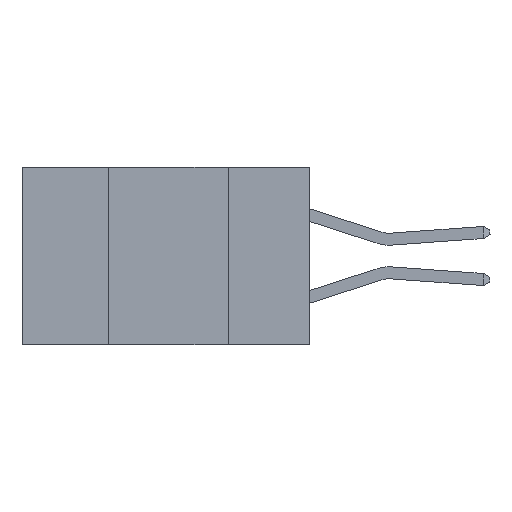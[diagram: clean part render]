
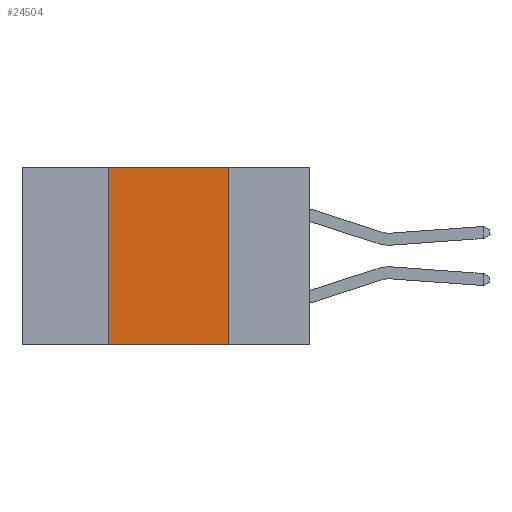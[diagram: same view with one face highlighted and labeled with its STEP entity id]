
A CAD part, left-side view. The second image highlights one B-rep face of the part: STEP entity #24504.
In plain terms, the highlighted planar face has unit normal (-1, 0, 0).
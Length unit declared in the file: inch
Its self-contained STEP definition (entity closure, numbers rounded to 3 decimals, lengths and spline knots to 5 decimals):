
#2264 = CARTESIAN_POINT ( 'NONE',  ( 0., 0.17, -0.37 ) ) ;
#2955 = FACE_OUTER_BOUND ( 'NONE', #8184, .T. ) ;
#3680 = VERTEX_POINT ( 'NONE', #21268 ) ;
#4613 = LINE ( 'NONE', #9639, #26238 ) ;
#5525 = PLANE ( 'NONE',  #18120 ) ;
#5615 = DIRECTION ( 'NONE',  ( 1., 0., 0. ) ) ;
#5854 = VERTEX_POINT ( 'NONE', #12949 ) ;
#7232 = DIRECTION ( 'NONE',  ( 0., -1., 0. ) ) ;
#7438 = ORIENTED_EDGE ( 'NONE', *, *, #27174, .T. ) ;
#7776 = EDGE_CURVE ( 'NONE', #5854, #3680, #4613, .T. ) ;
#8184 = EDGE_LOOP ( 'NONE', ( #24159, #22562, #12964, #7438 ) ) ;
#8770 = CARTESIAN_POINT ( 'NONE',  ( 0., 0.17, 0. ) ) ;
#9639 = CARTESIAN_POINT ( 'NONE',  ( 0., 0.42, -0.37 ) ) ;
#12634 = LINE ( 'NONE', #25622, #23812 ) ;
#12949 = CARTESIAN_POINT ( 'NONE',  ( 0., 0.42, -0.37 ) ) ;
#12964 = ORIENTED_EDGE ( 'NONE', *, *, #7776, .F. ) ;
#12987 = LINE ( 'NONE', #21781, #23513 ) ;
#14763 = VECTOR ( 'NONE', #7232, 39.37008 ) ;
#15152 = DIRECTION ( 'NONE',  ( 0., 0., -1. ) ) ;
#15993 = EDGE_CURVE ( 'NONE', #3680, #23481, #25927, .T. ) ;
#16129 = DIRECTION ( 'NONE',  ( 0., 0., 1. ) ) ;
#18120 = AXIS2_PLACEMENT_3D ( 'NONE', #26494, #5615, #20287 ) ;
#18886 = VERTEX_POINT ( 'NONE', #2264 ) ;
#19006 = EDGE_CURVE ( 'NONE', #23481, #18886, #12634, .T. ) ;
#20287 = DIRECTION ( 'NONE',  ( 0., 0., -1. ) ) ;
#21268 = CARTESIAN_POINT ( 'NONE',  ( 0., 0.42, 0. ) ) ;
#21781 = CARTESIAN_POINT ( 'NONE',  ( 0., 0.6, -0.37 ) ) ;
#21898 = CARTESIAN_POINT ( 'NONE',  ( 0., 0.6, 0. ) ) ;
#22562 = ORIENTED_EDGE ( 'NONE', *, *, #15993, .F. ) ;
#23481 = VERTEX_POINT ( 'NONE', #8770 ) ;
#23513 = VECTOR ( 'NONE', #23899, 39.37008 ) ;
#23812 = VECTOR ( 'NONE', #15152, 39.37008 ) ;
#23899 = DIRECTION ( 'NONE',  ( 0., -1., 0. ) ) ;
#24159 = ORIENTED_EDGE ( 'NONE', *, *, #19006, .F. ) ;
#24504 = ADVANCED_FACE ( 'NONE', ( #2955 ), #5525, .F. ) ;
#25622 = CARTESIAN_POINT ( 'NONE',  ( 0., 0.17, -0.37 ) ) ;
#25927 = LINE ( 'NONE', #21898, #14763 ) ;
#26238 = VECTOR ( 'NONE', #16129, 39.37008 ) ;
#26494 = CARTESIAN_POINT ( 'NONE',  ( 0., 0.6, 0. ) ) ;
#27174 = EDGE_CURVE ( 'NONE', #5854, #18886, #12987, .T. ) ;
